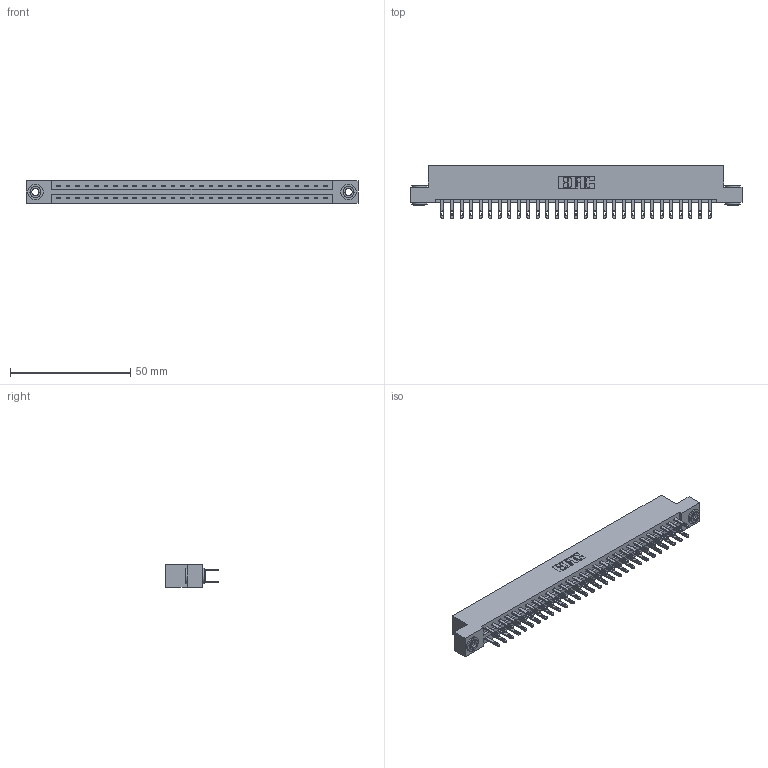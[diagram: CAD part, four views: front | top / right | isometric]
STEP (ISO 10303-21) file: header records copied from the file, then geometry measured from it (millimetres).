
FILE_DESCRIPTION (( 'STEP AP203' ), '1' );
FILE_NAME ('887-058-500-203.STEP', '2020-09-21T01:52:46', ( '' ), ( '' ), 'SwSTEP 2.0', 'SolidWorks 2020', '' );
FILE_SCHEMA (( 'CONFIG_CONTROL_DESIGN' ));
Length unit declared in the file: inch
Products named in the file (4): 887-058-500-203; 345-250-002_345-250-002-102; 837 Part_Flush Mounting Lugs - 0.156 Dia-TH; 345-292-001_345-293-100
Assembly tree (61 placements, depth 2):
  887-058-500-203
    837 Part_Flush Mounting Lugs - 0.156 Dia-TH
    345-292-001_345-293-100  x58
    345-250-002_345-250-002-102  x2
Bounding box: 137.92 x 21.85 x 9.4 mm (x, y, z)
Volume: 14558.9 mm3; surface area: 17200.5 mm2
Topology: 61 solids, 61 shells, 3052 faces, 9261 edges, 6170 vertices
Faces by surface type: plane 1936, cylinder 1108, cone 8
Entity records: 24746 total; most frequent: CARTESIAN_POINT 4153, ORIENTED_EDGE 4082, DIRECTION 3591, EDGE_CURVE 2041, LINE 1885, VECTOR 1885, VERTEX_POINT 1358, AXIS2_PLACEMENT_3D 853
